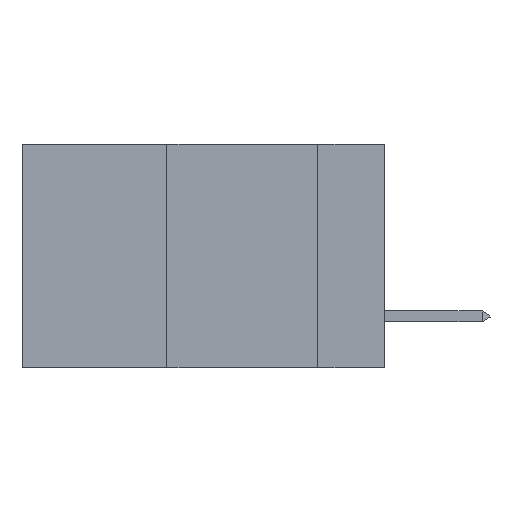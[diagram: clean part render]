
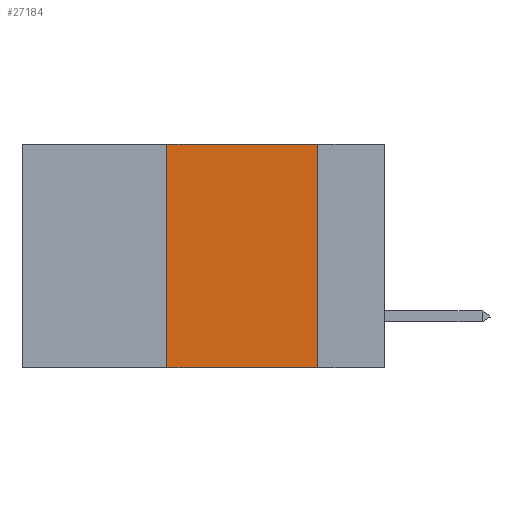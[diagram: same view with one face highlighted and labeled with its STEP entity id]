
A CAD part, left-side view. The second image highlights one B-rep face of the part: STEP entity #27184.
In plain terms, the highlighted planar face has unit normal (-1, 0, 0).
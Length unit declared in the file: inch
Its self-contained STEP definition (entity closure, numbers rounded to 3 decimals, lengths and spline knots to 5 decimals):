
#143 = VECTOR ( 'NONE', #7643, 39.37008 ) ;
#1258 = CARTESIAN_POINT ( 'NONE',  ( 0., 0.11, 0. ) ) ;
#2235 = ORIENTED_EDGE ( 'NONE', *, *, #23031, .F. ) ;
#2632 = DIRECTION ( 'NONE',  ( 0., -1., 0. ) ) ;
#3182 = LINE ( 'NONE', #18825, #143 ) ;
#3415 = VERTEX_POINT ( 'NONE', #3625 ) ;
#3625 = CARTESIAN_POINT ( 'NONE',  ( 0., 0.11, 0. ) ) ;
#4095 = PLANE ( 'NONE',  #16103 ) ;
#4108 = CARTESIAN_POINT ( 'NONE',  ( 0., 0.11, -0.37 ) ) ;
#4226 = VECTOR ( 'NONE', #25849, 39.37008 ) ;
#4354 = ORIENTED_EDGE ( 'NONE', *, *, #10179, .T. ) ;
#7643 = DIRECTION ( 'NONE',  ( 0., 0., 1. ) ) ;
#7648 = DIRECTION ( 'NONE',  ( 0., -1., 0. ) ) ;
#7906 = FACE_OUTER_BOUND ( 'NONE', #10613, .T. ) ;
#8671 = VERTEX_POINT ( 'NONE', #4108 ) ;
#10054 = ORIENTED_EDGE ( 'NONE', *, *, #22602, .F. ) ;
#10179 = EDGE_CURVE ( 'NONE', #23932, #8671, #18085, .T. ) ;
#10613 = EDGE_LOOP ( 'NONE', ( #14788, #2235, #10054, #4354 ) ) ;
#11220 = CARTESIAN_POINT ( 'NONE',  ( 0., 0.6, 0. ) ) ;
#11337 = CARTESIAN_POINT ( 'NONE',  ( 0., 0.6, 0. ) ) ;
#11903 = CARTESIAN_POINT ( 'NONE',  ( 0., 0.6, -0.37 ) ) ;
#14788 = ORIENTED_EDGE ( 'NONE', *, *, #16919, .F. ) ;
#16103 = AXIS2_PLACEMENT_3D ( 'NONE', #11337, #21606, #17979 ) ;
#16617 = VERTEX_POINT ( 'NONE', #27944 ) ;
#16919 = EDGE_CURVE ( 'NONE', #3415, #8671, #17816, .T. ) ;
#17816 = LINE ( 'NONE', #1258, #4226 ) ;
#17979 = DIRECTION ( 'NONE',  ( 0., 0., -1. ) ) ;
#18085 = LINE ( 'NONE', #11903, #20773 ) ;
#18825 = CARTESIAN_POINT ( 'NONE',  ( 0., 0.36, 0. ) ) ;
#20773 = VECTOR ( 'NONE', #7648, 39.37008 ) ;
#21606 = DIRECTION ( 'NONE',  ( 1., 0., 0. ) ) ;
#22602 = EDGE_CURVE ( 'NONE', #23932, #16617, #3182, .T. ) ;
#23031 = EDGE_CURVE ( 'NONE', #16617, #3415, #26145, .T. ) ;
#23748 = VECTOR ( 'NONE', #2632, 39.37008 ) ;
#23932 = VERTEX_POINT ( 'NONE', #27023 ) ;
#25849 = DIRECTION ( 'NONE',  ( 0., 0., -1. ) ) ;
#26145 = LINE ( 'NONE', #11220, #23748 ) ;
#27023 = CARTESIAN_POINT ( 'NONE',  ( 0., 0.36, -0.37 ) ) ;
#27184 = ADVANCED_FACE ( 'NONE', ( #7906 ), #4095, .F. ) ;
#27944 = CARTESIAN_POINT ( 'NONE',  ( 0., 0.36, 0. ) ) ;
